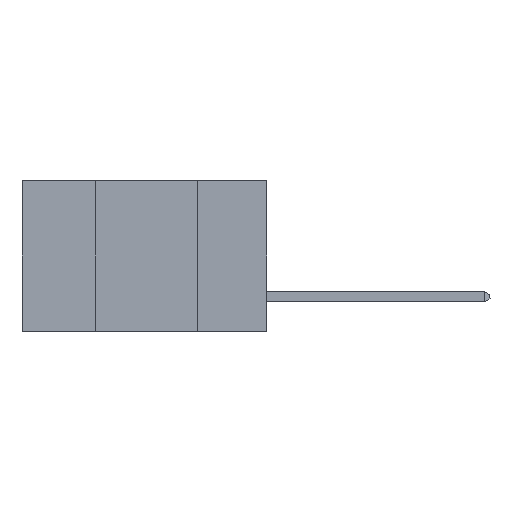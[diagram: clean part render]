
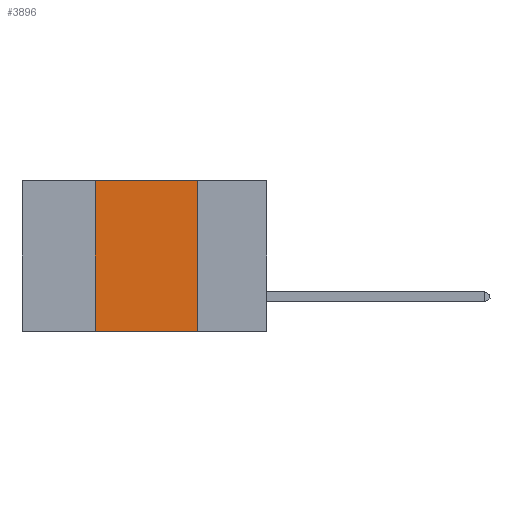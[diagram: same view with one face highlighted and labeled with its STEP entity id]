
A CAD part, left-side view. The second image highlights one B-rep face of the part: STEP entity #3896.
In plain terms, the highlighted planar face has unit normal (-1, 0, 0).
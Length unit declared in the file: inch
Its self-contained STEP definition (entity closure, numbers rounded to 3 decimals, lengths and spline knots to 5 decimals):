
#86 = CARTESIAN_POINT ( 'NONE',  ( 0., 0.17, 0. ) ) ;
#594 = VERTEX_POINT ( 'NONE', #13565 ) ;
#1088 = LINE ( 'NONE', #2106, #11942 ) ;
#1548 = VECTOR ( 'NONE', #7553, 39.37008 ) ;
#1603 = VERTEX_POINT ( 'NONE', #86 ) ;
#1750 = FACE_OUTER_BOUND ( 'NONE', #4410, .T. ) ;
#2106 = CARTESIAN_POINT ( 'NONE',  ( 0., 0.6, 0. ) ) ;
#2563 = CARTESIAN_POINT ( 'NONE',  ( 0., 0.42, 0. ) ) ;
#2622 = DIRECTION ( 'NONE',  ( 0., 0., 1. ) ) ;
#3755 = EDGE_CURVE ( 'NONE', #9414, #6050, #10341, .T. ) ;
#3856 = DIRECTION ( 'NONE',  ( 0., 0., -1. ) ) ;
#3896 = ADVANCED_FACE ( 'NONE', ( #1750 ), #12119, .F. ) ;
#4410 = EDGE_LOOP ( 'NONE', ( #4928, #12384, #5299, #5800 ) ) ;
#4928 = ORIENTED_EDGE ( 'NONE', *, *, #8366, .F. ) ;
#5299 = ORIENTED_EDGE ( 'NONE', *, *, #7794, .F. ) ;
#5800 = ORIENTED_EDGE ( 'NONE', *, *, #3755, .T. ) ;
#6050 = VERTEX_POINT ( 'NONE', #9565 ) ;
#6680 = VECTOR ( 'NONE', #13644, 39.37008 ) ;
#6779 = AXIS2_PLACEMENT_3D ( 'NONE', #13061, #10182, #3856 ) ;
#6994 = LINE ( 'NONE', #2563, #11993 ) ;
#7553 = DIRECTION ( 'NONE',  ( 0., -1., 0. ) ) ;
#7794 = EDGE_CURVE ( 'NONE', #9414, #594, #6994, .T. ) ;
#8366 = EDGE_CURVE ( 'NONE', #1603, #6050, #9992, .T. ) ;
#9296 = CARTESIAN_POINT ( 'NONE',  ( 0., 0.42, -0.37 ) ) ;
#9414 = VERTEX_POINT ( 'NONE', #9296 ) ;
#9565 = CARTESIAN_POINT ( 'NONE',  ( 0., 0.17, -0.37 ) ) ;
#9992 = LINE ( 'NONE', #13605, #6680 ) ;
#10182 = DIRECTION ( 'NONE',  ( 1., 0., 0. ) ) ;
#10341 = LINE ( 'NONE', #11540, #1548 ) ;
#10790 = DIRECTION ( 'NONE',  ( 0., -1., 0. ) ) ;
#11540 = CARTESIAN_POINT ( 'NONE',  ( 0., 0.6, -0.37 ) ) ;
#11942 = VECTOR ( 'NONE', #10790, 39.37008 ) ;
#11993 = VECTOR ( 'NONE', #2622, 39.37008 ) ;
#12119 = PLANE ( 'NONE',  #6779 ) ;
#12384 = ORIENTED_EDGE ( 'NONE', *, *, #13092, .F. ) ;
#13061 = CARTESIAN_POINT ( 'NONE',  ( 0., 0.6, 0. ) ) ;
#13092 = EDGE_CURVE ( 'NONE', #594, #1603, #1088, .T. ) ;
#13565 = CARTESIAN_POINT ( 'NONE',  ( 0., 0.42, 0. ) ) ;
#13605 = CARTESIAN_POINT ( 'NONE',  ( 0., 0.17, 0. ) ) ;
#13644 = DIRECTION ( 'NONE',  ( 0., 0., -1. ) ) ;
